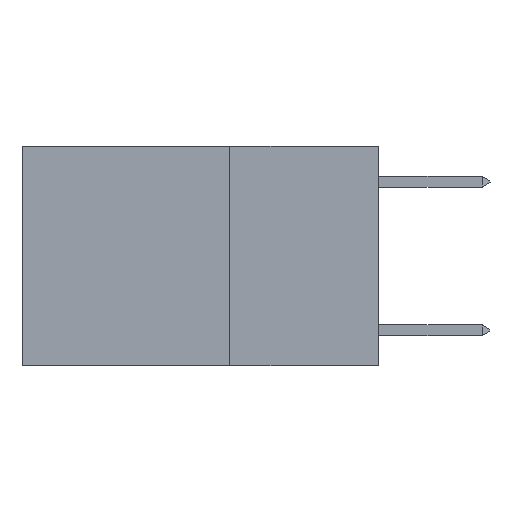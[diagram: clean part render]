
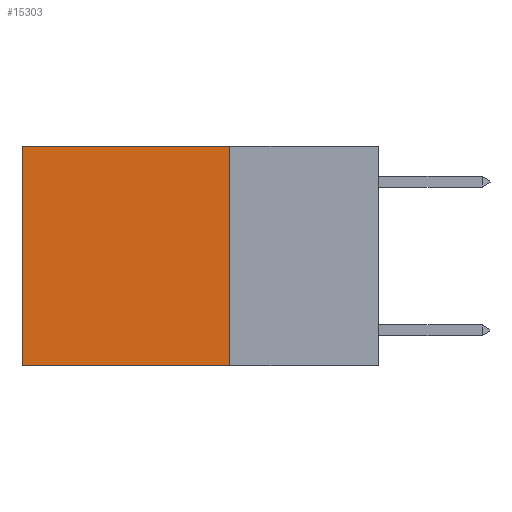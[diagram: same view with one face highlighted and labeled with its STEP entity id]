
A CAD part, left-side view. The second image highlights one B-rep face of the part: STEP entity #15303.
In plain terms, the highlighted planar face has unit normal (-1, 0, 0).
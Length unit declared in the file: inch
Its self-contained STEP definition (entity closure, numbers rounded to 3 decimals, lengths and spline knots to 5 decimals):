
#318 = EDGE_CURVE ( 'NONE', #22937, #1565, #19083, .T. ) ;
#458 = LINE ( 'NONE', #25804, #21254 ) ;
#524 = CARTESIAN_POINT ( 'NONE',  ( 0.2625, 0.25, 0. ) ) ;
#879 = AXIS2_PLACEMENT_3D ( 'NONE', #8598, #16667, #4618 ) ;
#1303 = EDGE_CURVE ( 'NONE', #12441, #5515, #4873, .T. ) ;
#1565 = VERTEX_POINT ( 'NONE', #4876 ) ;
#4618 = DIRECTION ( 'NONE',  ( 0., 0., -1. ) ) ;
#4873 = LINE ( 'NONE', #6031, #14948 ) ;
#4876 = CARTESIAN_POINT ( 'NONE',  ( 0.2625, 0.6, -0.37 ) ) ;
#5515 = VERTEX_POINT ( 'NONE', #8607 ) ;
#6031 = CARTESIAN_POINT ( 'NONE',  ( 0.2625, 0.25, 0. ) ) ;
#6954 = EDGE_LOOP ( 'NONE', ( #24849, #20574, #24975, #14181 ) ) ;
#8150 = DIRECTION ( 'NONE',  ( 0., 0., -1. ) ) ;
#8598 = CARTESIAN_POINT ( 'NONE',  ( 0.2625, 0.25, 0. ) ) ;
#8607 = CARTESIAN_POINT ( 'NONE',  ( 0.2625, 0.25, -0.37 ) ) ;
#9028 = DIRECTION ( 'NONE',  ( 0., 1., 0. ) ) ;
#9512 = EDGE_CURVE ( 'NONE', #5515, #1565, #25209, .T. ) ;
#9726 = CARTESIAN_POINT ( 'NONE',  ( 0.2625, 0.6, 0. ) ) ;
#11009 = DIRECTION ( 'NONE',  ( 0., 0., -1. ) ) ;
#12441 = VERTEX_POINT ( 'NONE', #524 ) ;
#13534 = CARTESIAN_POINT ( 'NONE',  ( 0.2625, 0.25, -0.37 ) ) ;
#14181 = ORIENTED_EDGE ( 'NONE', *, *, #21035, .T. ) ;
#14948 = VECTOR ( 'NONE', #8150, 39.37008 ) ;
#15303 = ADVANCED_FACE ( 'NONE', ( #18985 ), #17018, .F. ) ;
#16667 = DIRECTION ( 'NONE',  ( 1., 0., 0. ) ) ;
#17018 = PLANE ( 'NONE',  #879 ) ;
#17119 = VECTOR ( 'NONE', #9028, 39.37008 ) ;
#18985 = FACE_OUTER_BOUND ( 'NONE', #6954, .T. ) ;
#19083 = LINE ( 'NONE', #22927, #20950 ) ;
#19976 = DIRECTION ( 'NONE',  ( 0., 1., 0. ) ) ;
#20574 = ORIENTED_EDGE ( 'NONE', *, *, #9512, .F. ) ;
#20950 = VECTOR ( 'NONE', #11009, 39.37008 ) ;
#21035 = EDGE_CURVE ( 'NONE', #12441, #22937, #458, .T. ) ;
#21254 = VECTOR ( 'NONE', #19976, 39.37008 ) ;
#22927 = CARTESIAN_POINT ( 'NONE',  ( 0.2625, 0.6, 0. ) ) ;
#22937 = VERTEX_POINT ( 'NONE', #9726 ) ;
#24849 = ORIENTED_EDGE ( 'NONE', *, *, #318, .T. ) ;
#24975 = ORIENTED_EDGE ( 'NONE', *, *, #1303, .F. ) ;
#25209 = LINE ( 'NONE', #13534, #17119 ) ;
#25804 = CARTESIAN_POINT ( 'NONE',  ( 0.2625, 0.25, 0. ) ) ;
